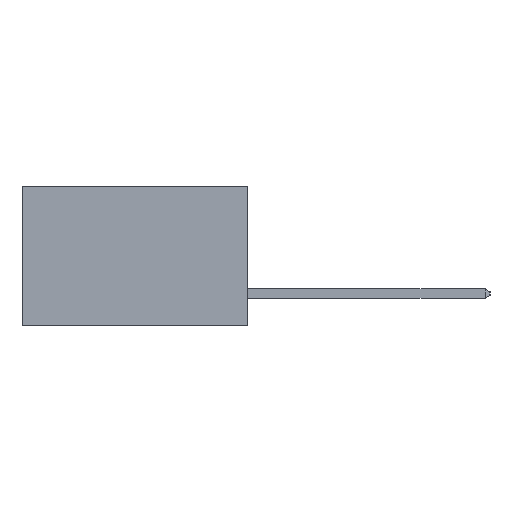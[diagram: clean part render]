
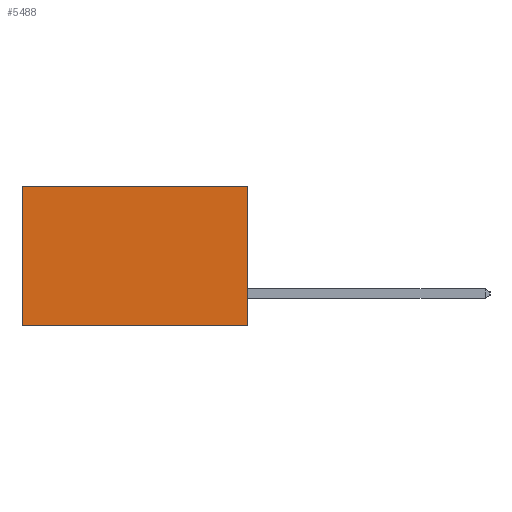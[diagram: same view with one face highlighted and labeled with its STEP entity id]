
A CAD part, left-side view. The second image highlights one B-rep face of the part: STEP entity #5488.
In plain terms, the highlighted planar face has unit normal (-1, 0, 0).
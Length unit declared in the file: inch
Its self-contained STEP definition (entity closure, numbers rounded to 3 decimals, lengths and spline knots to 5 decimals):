
#42 = DIRECTION ( 'NONE',  ( 0., 1., 0. ) ) ;
#1444 = VECTOR ( 'NONE', #4627, 39.37008 ) ;
#1503 = CARTESIAN_POINT ( 'NONE',  ( 0.298, 0.6, -0.37 ) ) ;
#1741 = VERTEX_POINT ( 'NONE', #4979 ) ;
#1896 = EDGE_LOOP ( 'NONE', ( #12201, #13932, #10367, #13577 ) ) ;
#2330 = EDGE_CURVE ( 'NONE', #7788, #4435, #9776, .T. ) ;
#3270 = VECTOR ( 'NONE', #12555, 39.37008 ) ;
#4435 = VERTEX_POINT ( 'NONE', #1503 ) ;
#4627 = DIRECTION ( 'NONE',  ( 0., 0., -1. ) ) ;
#4979 = CARTESIAN_POINT ( 'NONE',  ( 0.298, 0., 0. ) ) ;
#5161 = EDGE_CURVE ( 'NONE', #1741, #7788, #13991, .T. ) ;
#5488 = ADVANCED_FACE ( 'NONE', ( #7940 ), #5509, .F. ) ;
#5509 = PLANE ( 'NONE',  #11116 ) ;
#5744 = VECTOR ( 'NONE', #13843, 39.37008 ) ;
#5786 = VERTEX_POINT ( 'NONE', #7639 ) ;
#6790 = CARTESIAN_POINT ( 'NONE',  ( 0.298, 0., 0. ) ) ;
#7639 = CARTESIAN_POINT ( 'NONE',  ( 0.298, 0.6, 0. ) ) ;
#7788 = VERTEX_POINT ( 'NONE', #11851 ) ;
#7896 = DIRECTION ( 'NONE',  ( 0., 0., -1. ) ) ;
#7901 = DIRECTION ( 'NONE',  ( 1., 0., 0. ) ) ;
#7940 = FACE_OUTER_BOUND ( 'NONE', #1896, .T. ) ;
#8630 = CARTESIAN_POINT ( 'NONE',  ( 0.298, 0., 0. ) ) ;
#9324 = LINE ( 'NONE', #8630, #11746 ) ;
#9776 = LINE ( 'NONE', #11751, #3270 ) ;
#9890 = EDGE_CURVE ( 'NONE', #5786, #4435, #12151, .T. ) ;
#10367 = ORIENTED_EDGE ( 'NONE', *, *, #5161, .F. ) ;
#10909 = EDGE_CURVE ( 'NONE', #1741, #5786, #9324, .T. ) ;
#11116 = AXIS2_PLACEMENT_3D ( 'NONE', #15260, #7901, #7896 ) ;
#11746 = VECTOR ( 'NONE', #42, 39.37008 ) ;
#11751 = CARTESIAN_POINT ( 'NONE',  ( 0.298, 0., -0.37 ) ) ;
#11851 = CARTESIAN_POINT ( 'NONE',  ( 0.298, 0., -0.37 ) ) ;
#12151 = LINE ( 'NONE', #14915, #5744 ) ;
#12201 = ORIENTED_EDGE ( 'NONE', *, *, #9890, .T. ) ;
#12555 = DIRECTION ( 'NONE',  ( 0., 1., 0. ) ) ;
#13577 = ORIENTED_EDGE ( 'NONE', *, *, #10909, .T. ) ;
#13843 = DIRECTION ( 'NONE',  ( 0., 0., -1. ) ) ;
#13932 = ORIENTED_EDGE ( 'NONE', *, *, #2330, .F. ) ;
#13991 = LINE ( 'NONE', #6790, #1444 ) ;
#14915 = CARTESIAN_POINT ( 'NONE',  ( 0.298, 0.6, 0. ) ) ;
#15260 = CARTESIAN_POINT ( 'NONE',  ( 0.298, 0., 0. ) ) ;
